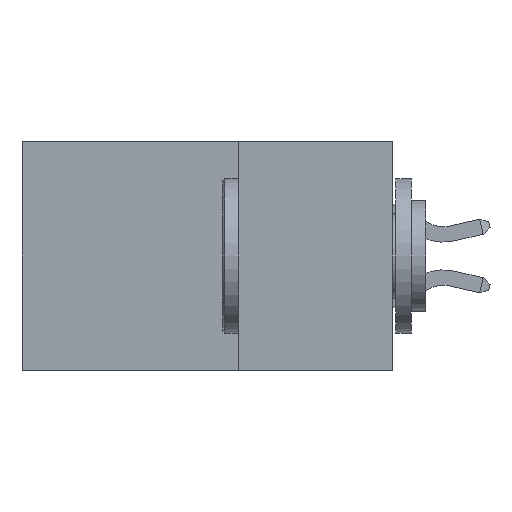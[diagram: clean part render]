
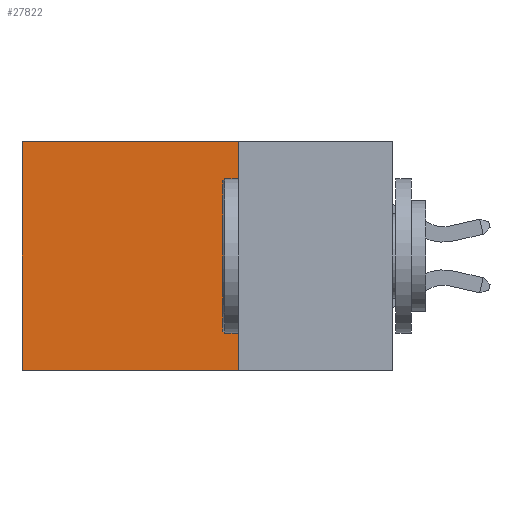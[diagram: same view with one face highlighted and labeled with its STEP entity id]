
A CAD part, left-side view. The second image highlights one B-rep face of the part: STEP entity #27822.
In plain terms, the highlighted planar face has unit normal (-1, 0, 0).
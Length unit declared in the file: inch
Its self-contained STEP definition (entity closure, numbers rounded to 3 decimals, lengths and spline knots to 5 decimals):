
#489 = LINE ( 'NONE', #5710, #20603 ) ;
#1465 = ORIENTED_EDGE ( 'NONE', *, *, #8307, .F. ) ;
#2480 = EDGE_LOOP ( 'NONE', ( #7441, #14966, #1465, #16861 ) ) ;
#3508 = VERTEX_POINT ( 'NONE', #17755 ) ;
#3608 = AXIS2_PLACEMENT_3D ( 'NONE', #22786, #7085, #25399 ) ;
#5710 = CARTESIAN_POINT ( 'NONE',  ( 0.2875, 0.6, 0. ) ) ;
#6089 = CARTESIAN_POINT ( 'NONE',  ( 0.2875, 0.25, 0. ) ) ;
#7005 = VECTOR ( 'NONE', #28977, 39.37008 ) ;
#7085 = DIRECTION ( 'NONE',  ( 1., 0., 0. ) ) ;
#7441 = ORIENTED_EDGE ( 'NONE', *, *, #14284, .T. ) ;
#8307 = EDGE_CURVE ( 'NONE', #12621, #31667, #27872, .T. ) ;
#8442 = DIRECTION ( 'NONE',  ( 0., 0., -1. ) ) ;
#9488 = CARTESIAN_POINT ( 'NONE',  ( 0.2875, 0.25, 0. ) ) ;
#11825 = VERTEX_POINT ( 'NONE', #24886 ) ;
#12397 = EDGE_CURVE ( 'NONE', #12621, #3508, #18677, .T. ) ;
#12621 = VERTEX_POINT ( 'NONE', #9488 ) ;
#13326 = CARTESIAN_POINT ( 'NONE',  ( 0.2875, 0.25, 0. ) ) ;
#13709 = CARTESIAN_POINT ( 'NONE',  ( 0.2875, 0.25, -0.37 ) ) ;
#14284 = EDGE_CURVE ( 'NONE', #3508, #11825, #489, .T. ) ;
#14966 = ORIENTED_EDGE ( 'NONE', *, *, #22281, .F. ) ;
#16861 = ORIENTED_EDGE ( 'NONE', *, *, #12397, .T. ) ;
#17755 = CARTESIAN_POINT ( 'NONE',  ( 0.2875, 0.6, 0. ) ) ;
#18677 = LINE ( 'NONE', #6089, #32511 ) ;
#18770 = LINE ( 'NONE', #13709, #31809 ) ;
#20603 = VECTOR ( 'NONE', #8442, 39.37008 ) ;
#22281 = EDGE_CURVE ( 'NONE', #31667, #11825, #18770, .T. ) ;
#22786 = CARTESIAN_POINT ( 'NONE',  ( 0.2875, 0.25, 0. ) ) ;
#23735 = FACE_OUTER_BOUND ( 'NONE', #2480, .T. ) ;
#24271 = DIRECTION ( 'NONE',  ( 0., 1., 0. ) ) ;
#24410 = DIRECTION ( 'NONE',  ( 0., 1., 0. ) ) ;
#24886 = CARTESIAN_POINT ( 'NONE',  ( 0.2875, 0.6, -0.37 ) ) ;
#25399 = DIRECTION ( 'NONE',  ( 0., 0., -1. ) ) ;
#27822 = ADVANCED_FACE ( 'NONE', ( #23735 ), #27888, .F. ) ;
#27872 = LINE ( 'NONE', #13326, #7005 ) ;
#27888 = PLANE ( 'NONE',  #3608 ) ;
#28977 = DIRECTION ( 'NONE',  ( 0., 0., -1. ) ) ;
#31667 = VERTEX_POINT ( 'NONE', #32909 ) ;
#31809 = VECTOR ( 'NONE', #24271, 39.37008 ) ;
#32511 = VECTOR ( 'NONE', #24410, 39.37008 ) ;
#32909 = CARTESIAN_POINT ( 'NONE',  ( 0.2875, 0.25, -0.37 ) ) ;
